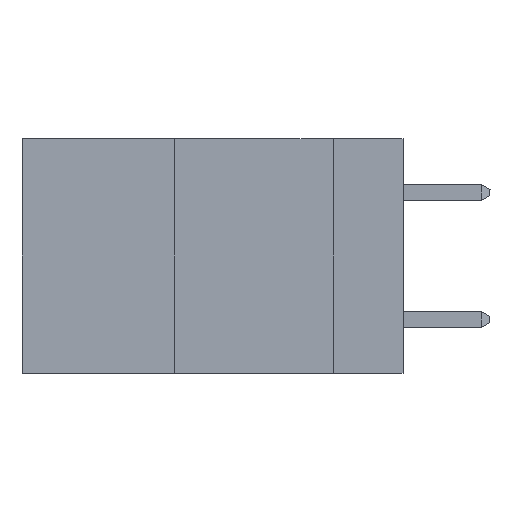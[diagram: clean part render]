
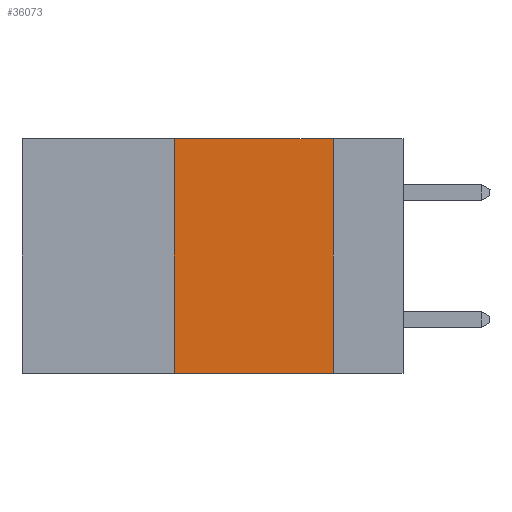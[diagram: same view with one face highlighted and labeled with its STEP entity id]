
A CAD part, left-side view. The second image highlights one B-rep face of the part: STEP entity #36073.
In plain terms, the highlighted planar face has unit normal (-1, 0, 0).
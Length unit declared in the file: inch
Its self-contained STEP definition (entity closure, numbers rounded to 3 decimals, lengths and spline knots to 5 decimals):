
#460 = AXIS2_PLACEMENT_3D ( 'NONE', #22914, #23109, #13642 ) ;
#1890 = FACE_OUTER_BOUND ( 'NONE', #13203, .T. ) ;
#4051 = LINE ( 'NONE', #28008, #9331 ) ;
#5402 = PLANE ( 'NONE',  #460 ) ;
#5764 = LINE ( 'NONE', #17760, #27908 ) ;
#7185 = CARTESIAN_POINT ( 'NONE',  ( 0., 0.36, -0.37 ) ) ;
#9331 = VECTOR ( 'NONE', #30576, 39.37008 ) ;
#11824 = EDGE_CURVE ( 'NONE', #36001, #13199, #5764, .T. ) ;
#11866 = DIRECTION ( 'NONE',  ( 0., 0., 1. ) ) ;
#11979 = ORIENTED_EDGE ( 'NONE', *, *, #11824, .F. ) ;
#13199 = VERTEX_POINT ( 'NONE', #29409 ) ;
#13203 = EDGE_LOOP ( 'NONE', ( #34336, #19603, #11979, #20483 ) ) ;
#13642 = DIRECTION ( 'NONE',  ( 0., 0., -1. ) ) ;
#13703 = CARTESIAN_POINT ( 'NONE',  ( 0., 0.11, -0.37 ) ) ;
#17760 = CARTESIAN_POINT ( 'NONE',  ( 0., 0.36, 0. ) ) ;
#19603 = ORIENTED_EDGE ( 'NONE', *, *, #23965, .F. ) ;
#20483 = ORIENTED_EDGE ( 'NONE', *, *, #37394, .T. ) ;
#20689 = DIRECTION ( 'NONE',  ( 0., 0., -1. ) ) ;
#21136 = VERTEX_POINT ( 'NONE', #13703 ) ;
#21794 = DIRECTION ( 'NONE',  ( 0., -1., 0. ) ) ;
#22914 = CARTESIAN_POINT ( 'NONE',  ( 0., 0.6, 0. ) ) ;
#23109 = DIRECTION ( 'NONE',  ( 1., 0., 0. ) ) ;
#23965 = EDGE_CURVE ( 'NONE', #13199, #27547, #4051, .T. ) ;
#24573 = LINE ( 'NONE', #36673, #35510 ) ;
#27547 = VERTEX_POINT ( 'NONE', #36440 ) ;
#27908 = VECTOR ( 'NONE', #11866, 39.37008 ) ;
#28008 = CARTESIAN_POINT ( 'NONE',  ( 0., 0.6, 0. ) ) ;
#29409 = CARTESIAN_POINT ( 'NONE',  ( 0., 0.36, 0. ) ) ;
#30576 = DIRECTION ( 'NONE',  ( 0., -1., 0. ) ) ;
#32440 = LINE ( 'NONE', #35761, #32857 ) ;
#32857 = VECTOR ( 'NONE', #20689, 39.37008 ) ;
#32941 = EDGE_CURVE ( 'NONE', #27547, #21136, #32440, .T. ) ;
#34336 = ORIENTED_EDGE ( 'NONE', *, *, #32941, .F. ) ;
#35510 = VECTOR ( 'NONE', #21794, 39.37008 ) ;
#35761 = CARTESIAN_POINT ( 'NONE',  ( 0., 0.11, 0. ) ) ;
#36001 = VERTEX_POINT ( 'NONE', #7185 ) ;
#36073 = ADVANCED_FACE ( 'NONE', ( #1890 ), #5402, .F. ) ;
#36440 = CARTESIAN_POINT ( 'NONE',  ( 0., 0.11, 0. ) ) ;
#36673 = CARTESIAN_POINT ( 'NONE',  ( 0., 0.6, -0.37 ) ) ;
#37394 = EDGE_CURVE ( 'NONE', #36001, #21136, #24573, .T. ) ;
